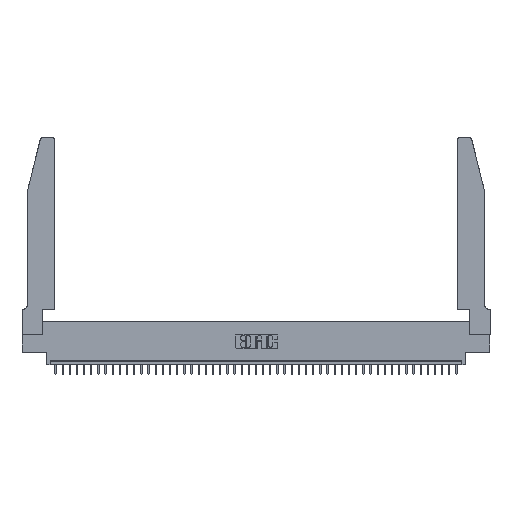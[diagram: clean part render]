
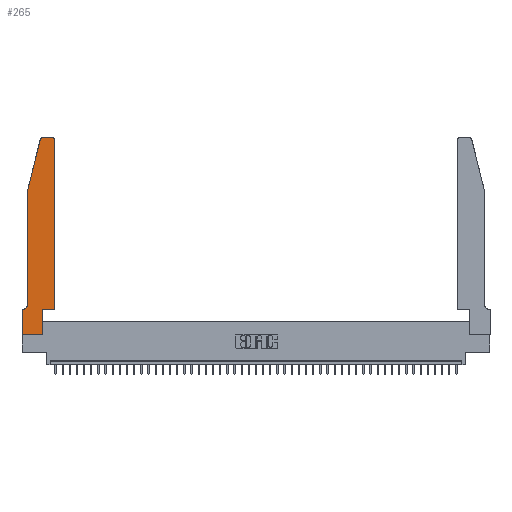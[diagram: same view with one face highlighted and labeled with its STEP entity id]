
A CAD part, top view. The second image highlights one B-rep face of the part: STEP entity #265.
In plain terms, the highlighted planar face has unit normal (0, 0, 1).
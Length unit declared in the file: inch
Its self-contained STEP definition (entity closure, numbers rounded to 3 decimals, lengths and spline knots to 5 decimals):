
#265 = ADVANCED_FACE ( 'NONE', ( #10885 ), #25466, .T. ) ;
#308 = CARTESIAN_POINT ( 'NONE',  ( 0.0755, 2., 0.37 ) ) ;
#328 = CARTESIAN_POINT ( 'NONE',  ( 0.2865, 0., 0.37 ) ) ;
#657 = AXIS2_PLACEMENT_3D ( 'NONE', #7211, #4162, #32035 ) ;
#875 = AXIS2_PLACEMENT_3D ( 'NONE', #10053, #31174, #31870 ) ;
#1244 = LINE ( 'NONE', #15399, #4050 ) ;
#1908 = ORIENTED_EDGE ( 'NONE', *, *, #37740, .T. ) ;
#2313 = CIRCLE ( 'NONE', #875, 0.07 ) ;
#2392 = VECTOR ( 'NONE', #11888, 39.37008 ) ;
#3425 = AXIS2_PLACEMENT_3D ( 'NONE', #43329, #32231, #21765 ) ;
#3938 = DIRECTION ( 'NONE',  ( 0., -1., 0. ) ) ;
#4050 = VECTOR ( 'NONE', #11011, 39.37008 ) ;
#4162 = DIRECTION ( 'NONE',  ( 0., 0., 1. ) ) ;
#4178 = VECTOR ( 'NONE', #13518, 39.37008 ) ;
#4637 = VERTEX_POINT ( 'NONE', #328 ) ;
#5423 = CARTESIAN_POINT ( 'NONE',  ( 0.0755, 2., 0.37 ) ) ;
#6874 = DIRECTION ( 'NONE',  ( -1., 0., 0. ) ) ;
#6916 = EDGE_CURVE ( 'NONE', #31045, #28082, #28850, .T. ) ;
#7211 = CARTESIAN_POINT ( 'NONE',  ( 0.4205, 2.72, 0.37 ) ) ;
#7481 = VERTEX_POINT ( 'NONE', #19492 ) ;
#8109 = VECTOR ( 'NONE', #13066, 39.37008 ) ;
#8431 = CARTESIAN_POINT ( 'NONE',  ( 0.284, 2.72, 0.37 ) ) ;
#9115 = ORIENTED_EDGE ( 'NONE', *, *, #29406, .T. ) ;
#9286 = CARTESIAN_POINT ( 'NONE',  ( 0., 0., 0.37 ) ) ;
#10053 = CARTESIAN_POINT ( 'NONE',  ( 0.0055, 0.42, 0.37 ) ) ;
#10241 = CARTESIAN_POINT ( 'NONE',  ( 0.4205, 2.75, 0.37 ) ) ;
#10816 = CARTESIAN_POINT ( 'NONE',  ( 0.0755, 0.35, 0.37 ) ) ;
#10885 = FACE_OUTER_BOUND ( 'NONE', #18250, .T. ) ;
#11011 = DIRECTION ( 'NONE',  ( 1., 0., 0. ) ) ;
#11063 = VECTOR ( 'NONE', #40235, 39.37008 ) ;
#11175 = DIRECTION ( 'NONE',  ( 1., 0., 0. ) ) ;
#11888 = DIRECTION ( 'NONE',  ( -0.239, -0.971, 0. ) ) ;
#12494 = ORIENTED_EDGE ( 'NONE', *, *, #17288, .T. ) ;
#13066 = DIRECTION ( 'NONE',  ( 0., 1., 0. ) ) ;
#13518 = DIRECTION ( 'NONE',  ( 0., -1., 0. ) ) ;
#13572 = VERTEX_POINT ( 'NONE', #28869 ) ;
#13639 = CARTESIAN_POINT ( 'NONE',  ( 0.2865, 0.35, 0.37 ) ) ;
#15399 = CARTESIAN_POINT ( 'NONE',  ( 0., 0., 0.37 ) ) ;
#16567 = LINE ( 'NONE', #17505, #8109 ) ;
#16654 = ORIENTED_EDGE ( 'NONE', *, *, #6916, .T. ) ;
#16898 = VERTEX_POINT ( 'NONE', #32823 ) ;
#17144 = VERTEX_POINT ( 'NONE', #9286 ) ;
#17288 = EDGE_CURVE ( 'NONE', #18957, #31045, #25090, .T. ) ;
#17505 = CARTESIAN_POINT ( 'NONE',  ( 0.2865, 0.35, 0.37 ) ) ;
#17887 = LINE ( 'NONE', #32033, #33412 ) ;
#18212 = VERTEX_POINT ( 'NONE', #18672 ) ;
#18250 = EDGE_LOOP ( 'NONE', ( #16654, #26007, #20872, #41406, #41291, #29691, #1908, #36637, #9115, #34749, #39873, #12494 ) ) ;
#18538 = EDGE_CURVE ( 'NONE', #13572, #7481, #2313, .T. ) ;
#18672 = CARTESIAN_POINT ( 'NONE',  ( 0., 0.35, 0.37 ) ) ;
#18957 = VERTEX_POINT ( 'NONE', #31345 ) ;
#19012 = VECTOR ( 'NONE', #6874, 39.37008 ) ;
#19492 = CARTESIAN_POINT ( 'NONE',  ( 0.0055, 0.35, 0.37 ) ) ;
#19783 = EDGE_CURVE ( 'NONE', #38509, #29220, #43680, .T. ) ;
#20872 = ORIENTED_EDGE ( 'NONE', *, *, #19783, .T. ) ;
#21765 = DIRECTION ( 'NONE',  ( 1., 0., 0. ) ) ;
#21888 = DIRECTION ( 'NONE',  ( -1., 0., 0. ) ) ;
#22248 = EDGE_CURVE ( 'NONE', #17144, #4637, #1244, .T. ) ;
#22607 = EDGE_CURVE ( 'NONE', #39315, #16898, #43185, .T. ) ;
#25090 = CIRCLE ( 'NONE', #657, 0.03 ) ;
#25156 = CARTESIAN_POINT ( 'NONE',  ( 0.2605, 2.75, 0.37 ) ) ;
#25466 = PLANE ( 'NONE',  #3425 ) ;
#25612 = EDGE_CURVE ( 'NONE', #28082, #38509, #36002, .T. ) ;
#25631 = LINE ( 'NONE', #10816, #19012 ) ;
#26007 = ORIENTED_EDGE ( 'NONE', *, *, #25612, .T. ) ;
#26060 = CARTESIAN_POINT ( 'NONE',  ( 0.284, 2.75, 0.37 ) ) ;
#26956 = DIRECTION ( 'NONE',  ( 1., 0., 0. ) ) ;
#28082 = VERTEX_POINT ( 'NONE', #26060 ) ;
#28850 = LINE ( 'NONE', #25156, #36383 ) ;
#28869 = CARTESIAN_POINT ( 'NONE',  ( 0.0755, 0.42, 0.37 ) ) ;
#29220 = VERTEX_POINT ( 'NONE', #5423 ) ;
#29249 = EDGE_CURVE ( 'NONE', #16898, #18957, #40460, .T. ) ;
#29406 = EDGE_CURVE ( 'NONE', #4637, #39315, #16567, .T. ) ;
#29691 = ORIENTED_EDGE ( 'NONE', *, *, #32526, .T. ) ;
#30767 = VECTOR ( 'NONE', #11175, 39.37008 ) ;
#31045 = VERTEX_POINT ( 'NONE', #10241 ) ;
#31174 = DIRECTION ( 'NONE',  ( 0., 0., -1. ) ) ;
#31345 = CARTESIAN_POINT ( 'NONE',  ( 0.4505, 2.72, 0.37 ) ) ;
#31870 = DIRECTION ( 'NONE',  ( -1., 0., 0. ) ) ;
#32033 = CARTESIAN_POINT ( 'NONE',  ( 0., 0., 0.37 ) ) ;
#32035 = DIRECTION ( 'NONE',  ( 1., 0., 0. ) ) ;
#32231 = DIRECTION ( 'NONE',  ( 0., 0., 1. ) ) ;
#32526 = EDGE_CURVE ( 'NONE', #7481, #18212, #25631, .T. ) ;
#32823 = CARTESIAN_POINT ( 'NONE',  ( 0.4505, 0.35, 0.37 ) ) ;
#33412 = VECTOR ( 'NONE', #3938, 39.37008 ) ;
#33777 = AXIS2_PLACEMENT_3D ( 'NONE', #8431, #44607, #26956 ) ;
#34749 = ORIENTED_EDGE ( 'NONE', *, *, #22607, .T. ) ;
#34882 = LINE ( 'NONE', #308, #4178 ) ;
#34935 = CARTESIAN_POINT ( 'NONE',  ( 0.25487, 2.72718, 0.37 ) ) ;
#36002 = CIRCLE ( 'NONE', #33777, 0.03 ) ;
#36383 = VECTOR ( 'NONE', #21888, 39.37008 ) ;
#36637 = ORIENTED_EDGE ( 'NONE', *, *, #22248, .T. ) ;
#36930 = CARTESIAN_POINT ( 'NONE',  ( 0.0755, 2., 0.37 ) ) ;
#37740 = EDGE_CURVE ( 'NONE', #18212, #17144, #17887, .T. ) ;
#38509 = VERTEX_POINT ( 'NONE', #34935 ) ;
#39315 = VERTEX_POINT ( 'NONE', #13639 ) ;
#39873 = ORIENTED_EDGE ( 'NONE', *, *, #29249, .T. ) ;
#40235 = DIRECTION ( 'NONE',  ( 0., 1., 0. ) ) ;
#40460 = LINE ( 'NONE', #43719, #11063 ) ;
#41291 = ORIENTED_EDGE ( 'NONE', *, *, #18538, .T. ) ;
#41406 = ORIENTED_EDGE ( 'NONE', *, *, #44312, .T. ) ;
#42751 = CARTESIAN_POINT ( 'NONE',  ( 0.4505, 0.35, 0.37 ) ) ;
#43185 = LINE ( 'NONE', #42751, #30767 ) ;
#43329 = CARTESIAN_POINT ( 'NONE',  ( 0., 0.35, 0.37 ) ) ;
#43680 = LINE ( 'NONE', #36930, #2392 ) ;
#43719 = CARTESIAN_POINT ( 'NONE',  ( 0.4505, 0.35, 0.37 ) ) ;
#44312 = EDGE_CURVE ( 'NONE', #29220, #13572, #34882, .T. ) ;
#44607 = DIRECTION ( 'NONE',  ( 0., 0., 1. ) ) ;
